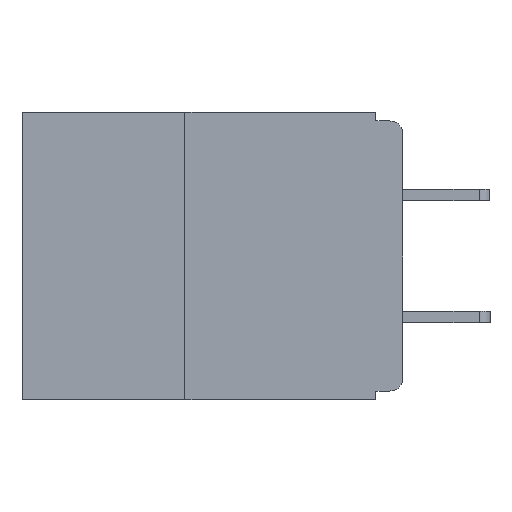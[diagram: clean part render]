
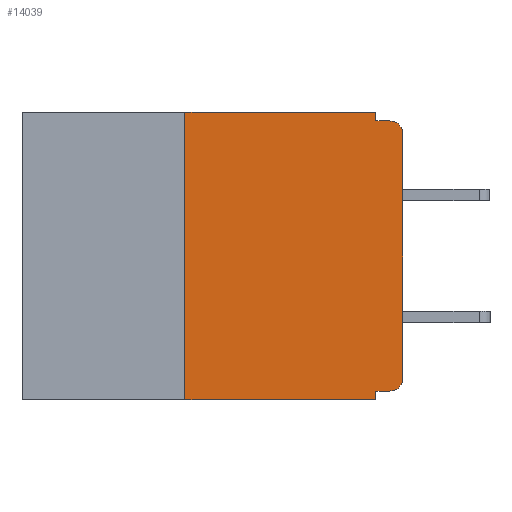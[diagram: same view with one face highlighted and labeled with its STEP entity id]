
A CAD part, left-side view. The second image highlights one B-rep face of the part: STEP entity #14039.
In plain terms, the highlighted planar face has unit normal (-1, 0, 0).
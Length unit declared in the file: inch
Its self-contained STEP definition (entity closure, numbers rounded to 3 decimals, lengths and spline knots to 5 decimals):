
#381 = EDGE_CURVE ( 'NONE', #7187, #1853, #3360, .T. ) ;
#791 = DIRECTION ( 'NONE',  ( 0., 1., 0. ) ) ;
#1047 = CARTESIAN_POINT ( 'NONE',  ( 0., 0.25, 0. ) ) ;
#1264 = CARTESIAN_POINT ( 'NONE',  ( 0., 0.031, 0. ) ) ;
#1712 = VERTEX_POINT ( 'NONE', #11220 ) ;
#1853 = VERTEX_POINT ( 'NONE', #13914 ) ;
#1979 = ORIENTED_EDGE ( 'NONE', *, *, #11194, .T. ) ;
#2489 = VECTOR ( 'NONE', #14313, 39.37008 ) ;
#3028 = VERTEX_POINT ( 'NONE', #1047 ) ;
#3076 = CARTESIAN_POINT ( 'NONE',  ( 0., 0., -0.32 ) ) ;
#3239 = DIRECTION ( 'NONE',  ( 0., 0., -1. ) ) ;
#3360 = LINE ( 'NONE', #19539, #11456 ) ;
#3377 = CARTESIAN_POINT ( 'NONE',  ( 0., 0.015, -0.025 ) ) ;
#3873 = VERTEX_POINT ( 'NONE', #18994 ) ;
#4214 = AXIS2_PLACEMENT_3D ( 'NONE', #13802, #16004, #3239 ) ;
#4763 = VECTOR ( 'NONE', #5760, 39.37008 ) ;
#4818 = LINE ( 'NONE', #1264, #16086 ) ;
#5416 = VERTEX_POINT ( 'NONE', #9506 ) ;
#5596 = DIRECTION ( 'NONE',  ( 0., 0., -1. ) ) ;
#5760 = DIRECTION ( 'NONE',  ( 0., 0., 1. ) ) ;
#7148 = VECTOR ( 'NONE', #24870, 39.37008 ) ;
#7187 = VERTEX_POINT ( 'NONE', #21919 ) ;
#8042 = LINE ( 'NONE', #3076, #23898 ) ;
#8072 = LINE ( 'NONE', #21094, #12985 ) ;
#8221 = ORIENTED_EDGE ( 'NONE', *, *, #11042, .T. ) ;
#8714 = ORIENTED_EDGE ( 'NONE', *, *, #19576, .F. ) ;
#9506 = CARTESIAN_POINT ( 'NONE',  ( 0., 0.031, 0. ) ) ;
#9635 = AXIS2_PLACEMENT_3D ( 'NONE', #10601, #24998, #12681 ) ;
#9811 = ORIENTED_EDGE ( 'NONE', *, *, #16794, .T. ) ;
#9962 = EDGE_CURVE ( 'NONE', #3873, #14601, #8072, .T. ) ;
#10317 = VECTOR ( 'NONE', #17433, 39.37008 ) ;
#10482 = CARTESIAN_POINT ( 'NONE',  ( 0., 0.437, 0. ) ) ;
#10504 = LINE ( 'NONE', #22320, #4763 ) ;
#10601 = CARTESIAN_POINT ( 'NONE',  ( 0., 0.015, -0.305 ) ) ;
#10757 = DIRECTION ( 'NONE',  ( 0., 0., -1. ) ) ;
#11025 = ORIENTED_EDGE ( 'NONE', *, *, #9962, .F. ) ;
#11042 = EDGE_CURVE ( 'NONE', #1712, #11932, #19464, .T. ) ;
#11194 = EDGE_CURVE ( 'NONE', #14841, #1712, #22318, .T. ) ;
#11220 = CARTESIAN_POINT ( 'NONE',  ( 0., 0., -0.305 ) ) ;
#11352 = EDGE_CURVE ( 'NONE', #23619, #14601, #15839, .T. ) ;
#11456 = VECTOR ( 'NONE', #20033, 39.37008 ) ;
#11499 = ORIENTED_EDGE ( 'NONE', *, *, #11352, .T. ) ;
#11847 = ORIENTED_EDGE ( 'NONE', *, *, #14118, .F. ) ;
#11932 = VERTEX_POINT ( 'NONE', #23116 ) ;
#12681 = DIRECTION ( 'NONE',  ( 0., 0., -1. ) ) ;
#12985 = VECTOR ( 'NONE', #10757, 39.37008 ) ;
#13802 = CARTESIAN_POINT ( 'NONE',  ( 0., 0.437, 0. ) ) ;
#13885 = PLANE ( 'NONE',  #4214 ) ;
#13914 = CARTESIAN_POINT ( 'NONE',  ( 0., 0.015, -0.01 ) ) ;
#14039 = ADVANCED_FACE ( 'NONE', ( #24036 ), #13885, .F. ) ;
#14118 = EDGE_CURVE ( 'NONE', #23619, #3028, #10504, .T. ) ;
#14313 = DIRECTION ( 'NONE',  ( 0., 0., 1. ) ) ;
#14601 = VERTEX_POINT ( 'NONE', #19617 ) ;
#14841 = VERTEX_POINT ( 'NONE', #18235 ) ;
#15522 = EDGE_CURVE ( 'NONE', #5416, #7187, #4818, .T. ) ;
#15839 = LINE ( 'NONE', #23495, #10317 ) ;
#16004 = DIRECTION ( 'NONE',  ( 1., 0., 0. ) ) ;
#16086 = VECTOR ( 'NONE', #16266, 39.37008 ) ;
#16266 = DIRECTION ( 'NONE',  ( 0., 0., -1. ) ) ;
#16794 = EDGE_CURVE ( 'NONE', #11932, #1853, #17982, .T. ) ;
#17433 = DIRECTION ( 'NONE',  ( 0., -1., 0. ) ) ;
#17982 = CIRCLE ( 'NONE', #21195, 0.015 ) ;
#18229 = DIRECTION ( 'NONE',  ( -1., 0., 0. ) ) ;
#18235 = CARTESIAN_POINT ( 'NONE',  ( 0., 0.015, -0.32 ) ) ;
#18994 = CARTESIAN_POINT ( 'NONE',  ( 0., 0.031, -0.32 ) ) ;
#19464 = LINE ( 'NONE', #26577, #2489 ) ;
#19539 = CARTESIAN_POINT ( 'NONE',  ( 0., 0., -0.01 ) ) ;
#19576 = EDGE_CURVE ( 'NONE', #14841, #3873, #8042, .T. ) ;
#19617 = CARTESIAN_POINT ( 'NONE',  ( 0., 0.031, -0.33 ) ) ;
#20033 = DIRECTION ( 'NONE',  ( 0., -1., 0. ) ) ;
#21094 = CARTESIAN_POINT ( 'NONE',  ( 0., 0.031, -0.33 ) ) ;
#21195 = AXIS2_PLACEMENT_3D ( 'NONE', #3377, #18229, #5596 ) ;
#21919 = CARTESIAN_POINT ( 'NONE',  ( 0., 0.031, -0.01 ) ) ;
#22318 = CIRCLE ( 'NONE', #9635, 0.015 ) ;
#22320 = CARTESIAN_POINT ( 'NONE',  ( 0., 0.25, -0.33 ) ) ;
#22502 = ORIENTED_EDGE ( 'NONE', *, *, #381, .F. ) ;
#23072 = LINE ( 'NONE', #10482, #7148 ) ;
#23116 = CARTESIAN_POINT ( 'NONE',  ( 0., 0., -0.025 ) ) ;
#23495 = CARTESIAN_POINT ( 'NONE',  ( 0., 0.437, -0.33 ) ) ;
#23619 = VERTEX_POINT ( 'NONE', #24989 ) ;
#23898 = VECTOR ( 'NONE', #791, 39.37008 ) ;
#24036 = FACE_OUTER_BOUND ( 'NONE', #27159, .T. ) ;
#24162 = EDGE_CURVE ( 'NONE', #3028, #5416, #23072, .T. ) ;
#24870 = DIRECTION ( 'NONE',  ( 0., -1., 0. ) ) ;
#24989 = CARTESIAN_POINT ( 'NONE',  ( 0., 0.25, -0.33 ) ) ;
#24998 = DIRECTION ( 'NONE',  ( -1., 0., 0. ) ) ;
#25466 = ORIENTED_EDGE ( 'NONE', *, *, #15522, .F. ) ;
#26023 = ORIENTED_EDGE ( 'NONE', *, *, #24162, .F. ) ;
#26577 = CARTESIAN_POINT ( 'NONE',  ( 0., 0., 0. ) ) ;
#27159 = EDGE_LOOP ( 'NONE', ( #8221, #9811, #22502, #25466, #26023, #11847, #11499, #11025, #8714, #1979 ) ) ;
